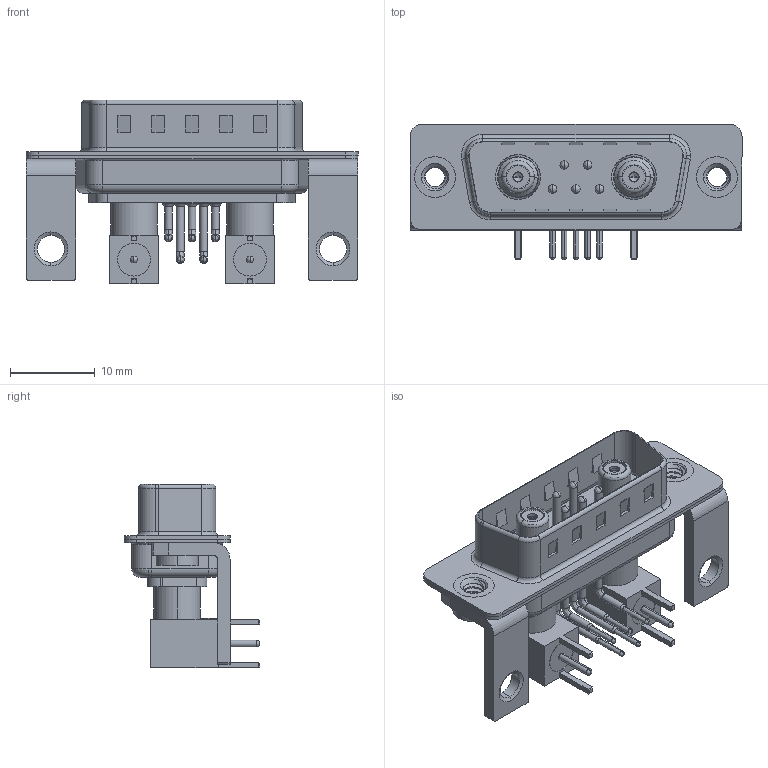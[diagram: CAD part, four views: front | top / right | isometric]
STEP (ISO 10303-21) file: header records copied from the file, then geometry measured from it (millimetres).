
FILE_DESCRIPTION (( 'STEP AP203' ), '1' );
FILE_NAME ('629-7W2-640-7TC.STEP', '2022-05-06T18:10:26', ( '' ), ( '' ), 'SwSTEP 2.0', 'SolidWorks 2020', '' );
FILE_SCHEMA (( 'CONFIG_CONTROL_DESIGN' ));
Length unit declared in the file: millimetre
Products named in the file (17): RA Back Shell; Co-Ax Jack Assy_RA; Insulator RA Pin; 629Combo Housing_7W2; Socket_RA; 629-7W2-640-7TC; 629Combo Stabilizer Bracket; Insulator Socket 2; Locking Collar; Co-Ax Jack_RA PC Tail; 629Combo Contact Row 2; 629Combo Contact Row 1; 629Combo Shell Front_15 Contacts; 629Combo Shell Rear_15 Contacts; 629Combo Threaded Rivet_2; Insulator Socket
Assembly tree (28 placements, depth 3):
  629-7W2-640-7TC
    629Combo Housing_7W2
    629Combo Shell Rear_15 Contacts
    629Combo Shell Front_15 Contacts
    629Combo Threaded Rivet_2  x2
    629Combo Stabilizer Bracket  x2
    Co-Ax Jack Assy_RA
      Co-Ax Jack_RA PC Tail
      Insulator Socket
      Insulator Socket 2
      Locking Collar
      Socket_RA
      RA Back Shell
      Insulator RA Pin
    Co-Ax Jack Assy_RA
      Co-Ax Jack_RA PC Tail
      Insulator Socket
      Insulator Socket 2
      Locking Collar
      Socket_RA
      RA Back Shell
      Insulator RA Pin
    629Combo Contact Row 1  x2
    629Combo Contact Row 2  x3
Bounding box: 39.2 x 16 x 21.71 mm (x, y, z)
Volume: 2762.7 mm3; surface area: 7425.4 mm2
Topology: 26 solids, 26 shells, 1242 faces, 3229 edges, 2062 vertices
Faces by surface type: plane 593, cylinder 471, cone 74, torus 62, bspline 38, sphere 4
Entity records: 26073 total; most frequent: CARTESIAN_POINT 5716, DIRECTION 3972, ORIENTED_EDGE 3706, EDGE_CURVE 1853, AXIS2_PLACEMENT_3D 1435, VERTEX_POINT 1189, LINE 1102, VECTOR 1102
